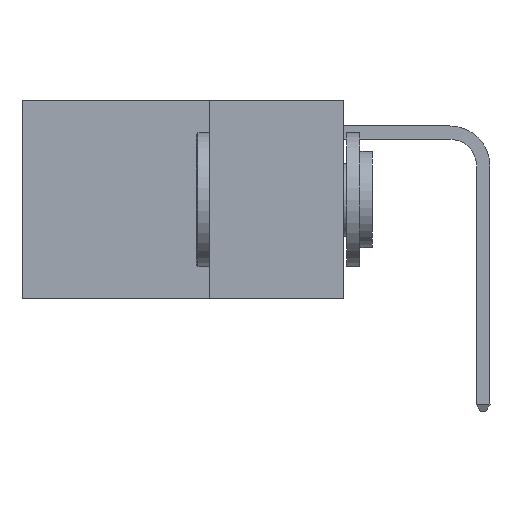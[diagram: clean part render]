
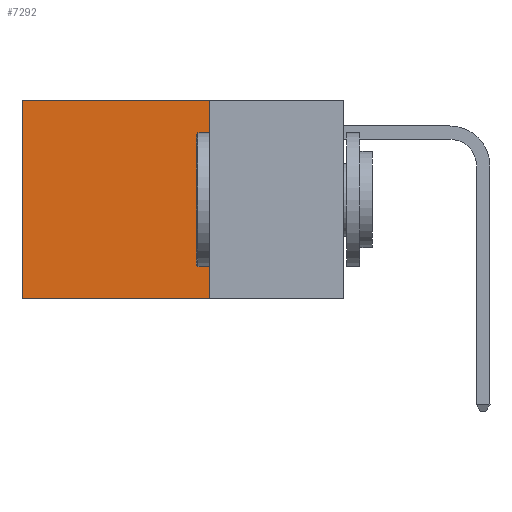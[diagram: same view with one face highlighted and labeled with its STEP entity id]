
A CAD part, left-side view. The second image highlights one B-rep face of the part: STEP entity #7292.
In plain terms, the highlighted planar face has unit normal (-1, 0, 0).
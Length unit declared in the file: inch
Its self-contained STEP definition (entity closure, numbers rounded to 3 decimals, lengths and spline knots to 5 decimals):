
#808 = CARTESIAN_POINT ( 'NONE',  ( 0.2625, 0.25, 0. ) ) ;
#1054 = EDGE_CURVE ( 'NONE', #6607, #16570, #2998, .T. ) ;
#1765 = CARTESIAN_POINT ( 'NONE',  ( 0.2625, 0.25, 0. ) ) ;
#2998 = LINE ( 'NONE', #808, #9671 ) ;
#3168 = CARTESIAN_POINT ( 'NONE',  ( 0.2625, 0.25, 0. ) ) ;
#3552 = VECTOR ( 'NONE', #15351, 39.37008 ) ;
#3582 = DIRECTION ( 'NONE',  ( 0., 0., -1. ) ) ;
#4173 = ORIENTED_EDGE ( 'NONE', *, *, #7135, .T. ) ;
#4990 = LINE ( 'NONE', #11151, #11588 ) ;
#5891 = DIRECTION ( 'NONE',  ( 1., 0., 0. ) ) ;
#6260 = CARTESIAN_POINT ( 'NONE',  ( 0.2625, 0.6, -0.37 ) ) ;
#6412 = CARTESIAN_POINT ( 'NONE',  ( 0.2625, 0.6, 0. ) ) ;
#6607 = VERTEX_POINT ( 'NONE', #1765 ) ;
#6881 = CARTESIAN_POINT ( 'NONE',  ( 0.2625, 0.6, 0. ) ) ;
#7135 = EDGE_CURVE ( 'NONE', #8838, #11928, #11907, .T. ) ;
#7292 = ADVANCED_FACE ( 'NONE', ( #12525 ), #13757, .F. ) ;
#7548 = LINE ( 'NONE', #11522, #3552 ) ;
#8420 = EDGE_LOOP ( 'NONE', ( #4173, #9138, #11737, #15036 ) ) ;
#8838 = VERTEX_POINT ( 'NONE', #6412 ) ;
#9138 = ORIENTED_EDGE ( 'NONE', *, *, #10419, .F. ) ;
#9671 = VECTOR ( 'NONE', #3582, 39.37008 ) ;
#9883 = CARTESIAN_POINT ( 'NONE',  ( 0.2625, 0.25, -0.37 ) ) ;
#10419 = EDGE_CURVE ( 'NONE', #16570, #11928, #4990, .T. ) ;
#11151 = CARTESIAN_POINT ( 'NONE',  ( 0.2625, 0.25, -0.37 ) ) ;
#11522 = CARTESIAN_POINT ( 'NONE',  ( 0.2625, 0.25, 0. ) ) ;
#11588 = VECTOR ( 'NONE', #13764, 39.37008 ) ;
#11737 = ORIENTED_EDGE ( 'NONE', *, *, #1054, .F. ) ;
#11907 = LINE ( 'NONE', #6881, #14942 ) ;
#11928 = VERTEX_POINT ( 'NONE', #6260 ) ;
#12525 = FACE_OUTER_BOUND ( 'NONE', #8420, .T. ) ;
#13405 = DIRECTION ( 'NONE',  ( 0., 0., -1. ) ) ;
#13757 = PLANE ( 'NONE',  #15703 ) ;
#13764 = DIRECTION ( 'NONE',  ( 0., 1., 0. ) ) ;
#14296 = EDGE_CURVE ( 'NONE', #6607, #8838, #7548, .T. ) ;
#14942 = VECTOR ( 'NONE', #13405, 39.37008 ) ;
#15034 = DIRECTION ( 'NONE',  ( 0., 0., -1. ) ) ;
#15036 = ORIENTED_EDGE ( 'NONE', *, *, #14296, .T. ) ;
#15351 = DIRECTION ( 'NONE',  ( 0., 1., 0. ) ) ;
#15703 = AXIS2_PLACEMENT_3D ( 'NONE', #3168, #5891, #15034 ) ;
#16570 = VERTEX_POINT ( 'NONE', #9883 ) ;
